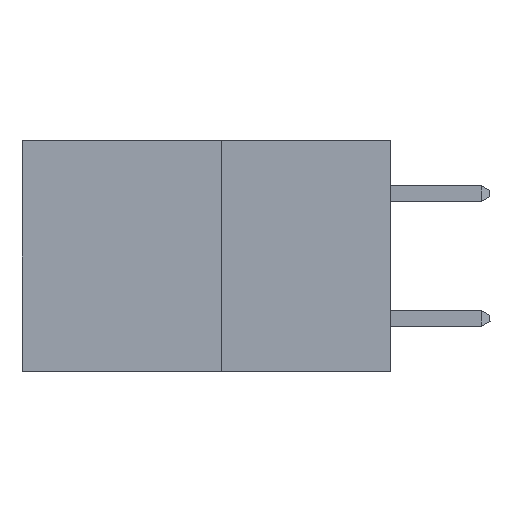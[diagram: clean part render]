
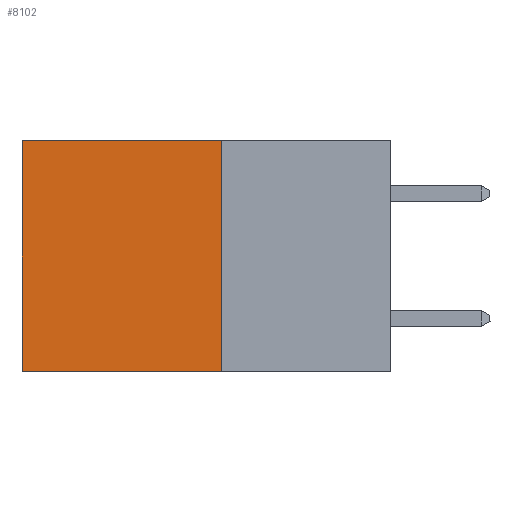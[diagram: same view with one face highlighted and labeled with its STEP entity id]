
A CAD part, left-side view. The second image highlights one B-rep face of the part: STEP entity #8102.
In plain terms, the highlighted planar face has unit normal (-1, 0, 0).
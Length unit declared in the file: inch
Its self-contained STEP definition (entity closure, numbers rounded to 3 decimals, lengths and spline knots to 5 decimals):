
#285 = CARTESIAN_POINT ( 'NONE',  ( 0.277, 0.27, 0. ) ) ;
#339 = ORIENTED_EDGE ( 'NONE', *, *, #1734, .F. ) ;
#444 = AXIS2_PLACEMENT_3D ( 'NONE', #11887, #11659, #11606 ) ;
#1137 = VERTEX_POINT ( 'NONE', #6343 ) ;
#1734 = EDGE_CURVE ( 'NONE', #1137, #19395, #15915, .T. ) ;
#2096 = VECTOR ( 'NONE', #12465, 39.37008 ) ;
#2308 = DIRECTION ( 'NONE',  ( 0., 0., -1. ) ) ;
#2937 = CARTESIAN_POINT ( 'NONE',  ( 0.277, 0.59, -0.37 ) ) ;
#3415 = EDGE_CURVE ( 'NONE', #3889, #15321, #10937, .T. ) ;
#3686 = VECTOR ( 'NONE', #10843, 39.37008 ) ;
#3889 = VERTEX_POINT ( 'NONE', #15226 ) ;
#6107 = DIRECTION ( 'NONE',  ( 0., 0., -1. ) ) ;
#6343 = CARTESIAN_POINT ( 'NONE',  ( 0.277, 0.27, 0. ) ) ;
#6847 = LINE ( 'NONE', #15924, #2096 ) ;
#7302 = ORIENTED_EDGE ( 'NONE', *, *, #17191, .T. ) ;
#7772 = VECTOR ( 'NONE', #6107, 39.37008 ) ;
#8102 = ADVANCED_FACE ( 'NONE', ( #16960 ), #12035, .F. ) ;
#9474 = CARTESIAN_POINT ( 'NONE',  ( 0.277, 0.27, -0.37 ) ) ;
#10843 = DIRECTION ( 'NONE',  ( 0., 1., 0. ) ) ;
#10937 = LINE ( 'NONE', #2937, #14452 ) ;
#11606 = DIRECTION ( 'NONE',  ( 0., 0., -1. ) ) ;
#11621 = ORIENTED_EDGE ( 'NONE', *, *, #3415, .T. ) ;
#11659 = DIRECTION ( 'NONE',  ( 1., 0., 0. ) ) ;
#11887 = CARTESIAN_POINT ( 'NONE',  ( 0.277, 0.27, -0.37 ) ) ;
#12035 = PLANE ( 'NONE',  #444 ) ;
#12465 = DIRECTION ( 'NONE',  ( 0., 1., 0. ) ) ;
#12567 = CARTESIAN_POINT ( 'NONE',  ( 0.277, 0.27, -0.37 ) ) ;
#13242 = ORIENTED_EDGE ( 'NONE', *, *, #15863, .F. ) ;
#14452 = VECTOR ( 'NONE', #2308, 39.37008 ) ;
#15226 = CARTESIAN_POINT ( 'NONE',  ( 0.277, 0.59, 0. ) ) ;
#15321 = VERTEX_POINT ( 'NONE', #18806 ) ;
#15863 = EDGE_CURVE ( 'NONE', #19395, #15321, #6847, .T. ) ;
#15915 = LINE ( 'NONE', #12567, #7772 ) ;
#15924 = CARTESIAN_POINT ( 'NONE',  ( 0.277, 0.27, -0.37 ) ) ;
#16960 = FACE_OUTER_BOUND ( 'NONE', #17159, .T. ) ;
#17159 = EDGE_LOOP ( 'NONE', ( #11621, #13242, #339, #7302 ) ) ;
#17191 = EDGE_CURVE ( 'NONE', #1137, #3889, #21075, .T. ) ;
#18806 = CARTESIAN_POINT ( 'NONE',  ( 0.277, 0.59, -0.37 ) ) ;
#19395 = VERTEX_POINT ( 'NONE', #9474 ) ;
#21075 = LINE ( 'NONE', #285, #3686 ) ;
